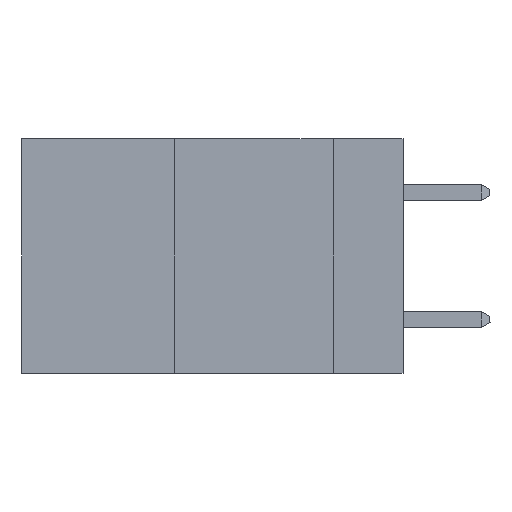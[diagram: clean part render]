
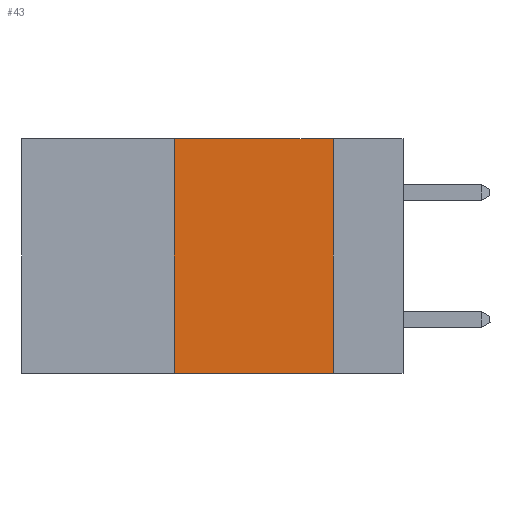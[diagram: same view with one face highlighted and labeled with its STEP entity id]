
A CAD part, left-side view. The second image highlights one B-rep face of the part: STEP entity #43.
In plain terms, the highlighted planar face has unit normal (-1, 0, 0).
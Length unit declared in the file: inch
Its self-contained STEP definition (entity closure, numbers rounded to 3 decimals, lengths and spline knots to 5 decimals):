
#43 = ADVANCED_FACE ( 'NONE', ( #13773 ), #9887, .F. ) ;
#1180 = EDGE_CURVE ( 'NONE', #6823, #2588, #9773, .T. ) ;
#2588 = VERTEX_POINT ( 'NONE', #21053 ) ;
#3053 = CARTESIAN_POINT ( 'NONE',  ( 0., 0.36, -0.37 ) ) ;
#3124 = EDGE_CURVE ( 'NONE', #2588, #7364, #21239, .T. ) ;
#4572 = ORIENTED_EDGE ( 'NONE', *, *, #13656, .T. ) ;
#4593 = CARTESIAN_POINT ( 'NONE',  ( 0., 0.11, 0. ) ) ;
#4885 = VECTOR ( 'NONE', #22482, 39.37008 ) ;
#5786 = DIRECTION ( 'NONE',  ( 1., 0., 0. ) ) ;
#6150 = EDGE_CURVE ( 'NONE', #7364, #8657, #22000, .T. ) ;
#6580 = ORIENTED_EDGE ( 'NONE', *, *, #6150, .F. ) ;
#6812 = VECTOR ( 'NONE', #8016, 39.37008 ) ;
#6823 = VERTEX_POINT ( 'NONE', #3053 ) ;
#7364 = VERTEX_POINT ( 'NONE', #4593 ) ;
#7775 = LINE ( 'NONE', #12166, #12615 ) ;
#8016 = DIRECTION ( 'NONE',  ( 0., -1., 0. ) ) ;
#8138 = DIRECTION ( 'NONE',  ( 0., 0., -1. ) ) ;
#8657 = VERTEX_POINT ( 'NONE', #17478 ) ;
#8871 = ORIENTED_EDGE ( 'NONE', *, *, #1180, .F. ) ;
#9390 = CARTESIAN_POINT ( 'NONE',  ( 0., 0.6, 0. ) ) ;
#9773 = LINE ( 'NONE', #20732, #4885 ) ;
#9887 = PLANE ( 'NONE',  #18098 ) ;
#12166 = CARTESIAN_POINT ( 'NONE',  ( 0., 0.6, -0.37 ) ) ;
#12279 = DIRECTION ( 'NONE',  ( 0., 0., -1. ) ) ;
#12615 = VECTOR ( 'NONE', #21147, 39.37008 ) ;
#13152 = ORIENTED_EDGE ( 'NONE', *, *, #3124, .F. ) ;
#13656 = EDGE_CURVE ( 'NONE', #6823, #8657, #7775, .T. ) ;
#13773 = FACE_OUTER_BOUND ( 'NONE', #22899, .T. ) ;
#17226 = VECTOR ( 'NONE', #12279, 39.37008 ) ;
#17478 = CARTESIAN_POINT ( 'NONE',  ( 0., 0.11, -0.37 ) ) ;
#18098 = AXIS2_PLACEMENT_3D ( 'NONE', #9390, #5786, #8138 ) ;
#18810 = CARTESIAN_POINT ( 'NONE',  ( 0., 0.6, 0. ) ) ;
#19433 = CARTESIAN_POINT ( 'NONE',  ( 0., 0.11, 0. ) ) ;
#20732 = CARTESIAN_POINT ( 'NONE',  ( 0., 0.36, 0. ) ) ;
#21053 = CARTESIAN_POINT ( 'NONE',  ( 0., 0.36, 0. ) ) ;
#21147 = DIRECTION ( 'NONE',  ( 0., -1., 0. ) ) ;
#21239 = LINE ( 'NONE', #18810, #6812 ) ;
#22000 = LINE ( 'NONE', #19433, #17226 ) ;
#22482 = DIRECTION ( 'NONE',  ( 0., 0., 1. ) ) ;
#22899 = EDGE_LOOP ( 'NONE', ( #6580, #13152, #8871, #4572 ) ) ;
